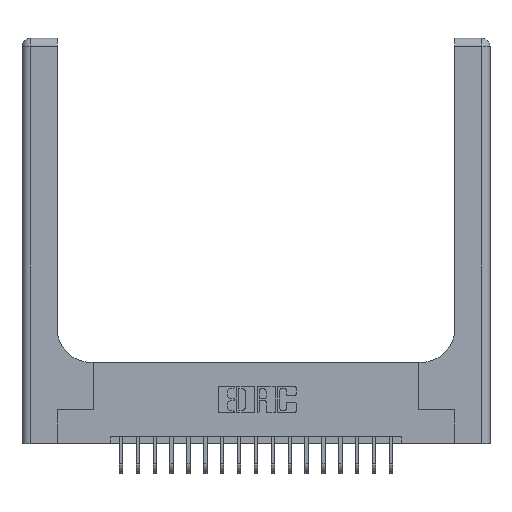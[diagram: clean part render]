
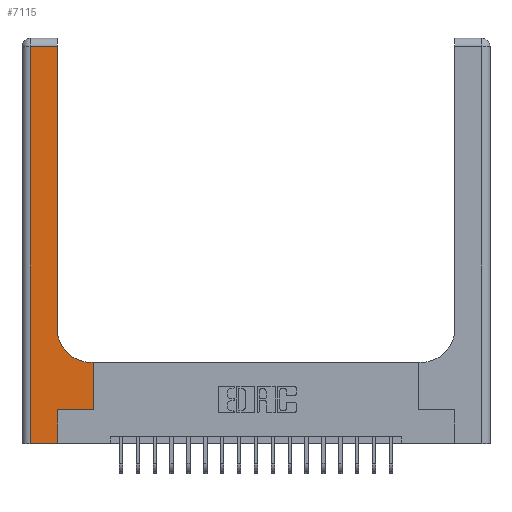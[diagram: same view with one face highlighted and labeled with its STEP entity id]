
A CAD part, top view. The second image highlights one B-rep face of the part: STEP entity #7115.
In plain terms, the highlighted planar face has unit normal (0, 0, 1).
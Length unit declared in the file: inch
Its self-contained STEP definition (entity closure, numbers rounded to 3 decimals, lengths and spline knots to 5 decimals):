
#13 = CARTESIAN_POINT ( 'NONE',  ( 0.06, 0., 0.37 ) ) ;
#46 = ORIENTED_EDGE ( 'NONE', *, *, #21421, .T. ) ;
#71 = CARTESIAN_POINT ( 'NONE',  ( 0.51, 0.85, 0.37 ) ) ;
#268 = VECTOR ( 'NONE', #19457, 39.37008 ) ;
#301 = EDGE_CURVE ( 'NONE', #13568, #17873, #3238, .T. ) ;
#465 = EDGE_CURVE ( 'NONE', #5518, #16317, #17064, .T. ) ;
#588 = DIRECTION ( 'NONE',  ( 0., 1., 0. ) ) ;
#1293 = VECTOR ( 'NONE', #14176, 39.37008 ) ;
#1464 = AXIS2_PLACEMENT_3D ( 'NONE', #3175, #21317, #6177 ) ;
#1629 = VECTOR ( 'NONE', #2019, 39.37008 ) ;
#2019 = DIRECTION ( 'NONE',  ( 0., 1., 0. ) ) ;
#2052 = ORIENTED_EDGE ( 'NONE', *, *, #13087, .T. ) ;
#2543 = AXIS2_PLACEMENT_3D ( 'NONE', #71, #15351, #6852 ) ;
#2748 = VECTOR ( 'NONE', #5671, 39.37008 ) ;
#2801 = EDGE_CURVE ( 'NONE', #16950, #19923, #12743, .T. ) ;
#3175 = CARTESIAN_POINT ( 'NONE',  ( 0., 3., 0.37 ) ) ;
#3238 = LINE ( 'NONE', #14969, #18581 ) ;
#3906 = CARTESIAN_POINT ( 'NONE',  ( 0.528, 0.25, 0.37 ) ) ;
#4281 = CARTESIAN_POINT ( 'NONE',  ( 0.51, 0.6, 0.37 ) ) ;
#4560 = CARTESIAN_POINT ( 'NONE',  ( 0.265, 0., 0.37 ) ) ;
#5459 = ORIENTED_EDGE ( 'NONE', *, *, #301, .T. ) ;
#5518 = VERTEX_POINT ( 'NONE', #18241 ) ;
#5563 = LINE ( 'NONE', #5785, #2748 ) ;
#5671 = DIRECTION ( 'NONE',  ( 1., 0., 0. ) ) ;
#5785 = CARTESIAN_POINT ( 'NONE',  ( 0., 0., 0.37 ) ) ;
#5808 = ORIENTED_EDGE ( 'NONE', *, *, #465, .T. ) ;
#5839 = ORIENTED_EDGE ( 'NONE', *, *, #2801, .T. ) ;
#6177 = DIRECTION ( 'NONE',  ( -1., 0., 0. ) ) ;
#6814 = CARTESIAN_POINT ( 'NONE',  ( 0.265, 0.25, 0.37 ) ) ;
#6852 = DIRECTION ( 'NONE',  ( 1., 0., 0. ) ) ;
#7031 = LINE ( 'NONE', #15197, #10544 ) ;
#7115 = ADVANCED_FACE ( 'NONE', ( #7844 ), #11387, .F. ) ;
#7195 = LINE ( 'NONE', #17691, #21712 ) ;
#7434 = CARTESIAN_POINT ( 'NONE',  ( 0.06, 3., 0.37 ) ) ;
#7844 = FACE_OUTER_BOUND ( 'NONE', #15691, .T. ) ;
#7966 = VERTEX_POINT ( 'NONE', #4560 ) ;
#8122 = VERTEX_POINT ( 'NONE', #18271 ) ;
#10544 = VECTOR ( 'NONE', #18519, 39.37008 ) ;
#10629 = EDGE_CURVE ( 'NONE', #16317, #16950, #7195, .T. ) ;
#10662 = ORIENTED_EDGE ( 'NONE', *, *, #19062, .T. ) ;
#11216 = CARTESIAN_POINT ( 'NONE',  ( 0.26, 2.94, 0.37 ) ) ;
#11387 = PLANE ( 'NONE',  #1464 ) ;
#12422 = LINE ( 'NONE', #20809, #1293 ) ;
#12743 = LINE ( 'NONE', #7434, #268 ) ;
#13087 = EDGE_CURVE ( 'NONE', #7966, #16704, #12422, .T. ) ;
#13568 = VERTEX_POINT ( 'NONE', #14262 ) ;
#13763 = CARTESIAN_POINT ( 'NONE',  ( 0.26, 3., 0.37 ) ) ;
#14176 = DIRECTION ( 'NONE',  ( 0., 1., 0. ) ) ;
#14262 = CARTESIAN_POINT ( 'NONE',  ( 0.528, 0.6, 0.37 ) ) ;
#14969 = CARTESIAN_POINT ( 'NONE',  ( 0.26, 0.6, 0.37 ) ) ;
#15197 = CARTESIAN_POINT ( 'NONE',  ( 0.265, 0.25, 0.37 ) ) ;
#15351 = DIRECTION ( 'NONE',  ( 0., 0., -1. ) ) ;
#15527 = EDGE_CURVE ( 'NONE', #16704, #8122, #7031, .T. ) ;
#15691 = EDGE_LOOP ( 'NONE', ( #5808, #19503, #5839, #19493, #2052, #15873, #46, #5459, #10662 ) ) ;
#15873 = ORIENTED_EDGE ( 'NONE', *, *, #15527, .T. ) ;
#16161 = EDGE_CURVE ( 'NONE', #19923, #7966, #5563, .T. ) ;
#16317 = VERTEX_POINT ( 'NONE', #11216 ) ;
#16704 = VERTEX_POINT ( 'NONE', #6814 ) ;
#16950 = VERTEX_POINT ( 'NONE', #17939 ) ;
#17064 = LINE ( 'NONE', #13763, #1629 ) ;
#17691 = CARTESIAN_POINT ( 'NONE',  ( 0., 2.94, 0.37 ) ) ;
#17873 = VERTEX_POINT ( 'NONE', #4281 ) ;
#17939 = CARTESIAN_POINT ( 'NONE',  ( 0.06, 2.94, 0.37 ) ) ;
#18241 = CARTESIAN_POINT ( 'NONE',  ( 0.26, 0.85, 0.37 ) ) ;
#18271 = CARTESIAN_POINT ( 'NONE',  ( 0.528, 0.25, 0.37 ) ) ;
#18519 = DIRECTION ( 'NONE',  ( 1., 0., 0. ) ) ;
#18581 = VECTOR ( 'NONE', #21605, 39.37008 ) ;
#19062 = EDGE_CURVE ( 'NONE', #17873, #5518, #19147, .T. ) ;
#19065 = LINE ( 'NONE', #3906, #19565 ) ;
#19147 = CIRCLE ( 'NONE', #2543, 0.25 ) ;
#19449 = DIRECTION ( 'NONE',  ( -1., 0., 0. ) ) ;
#19457 = DIRECTION ( 'NONE',  ( 0., -1., 0. ) ) ;
#19493 = ORIENTED_EDGE ( 'NONE', *, *, #16161, .T. ) ;
#19503 = ORIENTED_EDGE ( 'NONE', *, *, #10629, .T. ) ;
#19565 = VECTOR ( 'NONE', #588, 39.37008 ) ;
#19923 = VERTEX_POINT ( 'NONE', #13 ) ;
#20809 = CARTESIAN_POINT ( 'NONE',  ( 0.265, 0., 0.37 ) ) ;
#21317 = DIRECTION ( 'NONE',  ( 0., 0., -1. ) ) ;
#21421 = EDGE_CURVE ( 'NONE', #8122, #13568, #19065, .T. ) ;
#21605 = DIRECTION ( 'NONE',  ( -1., 0., 0. ) ) ;
#21712 = VECTOR ( 'NONE', #19449, 39.37008 ) ;
